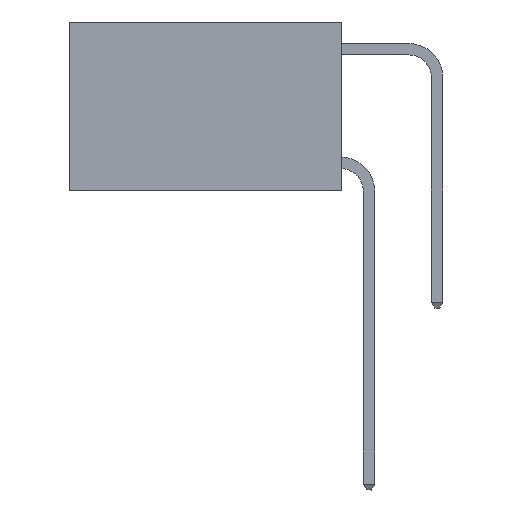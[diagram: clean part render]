
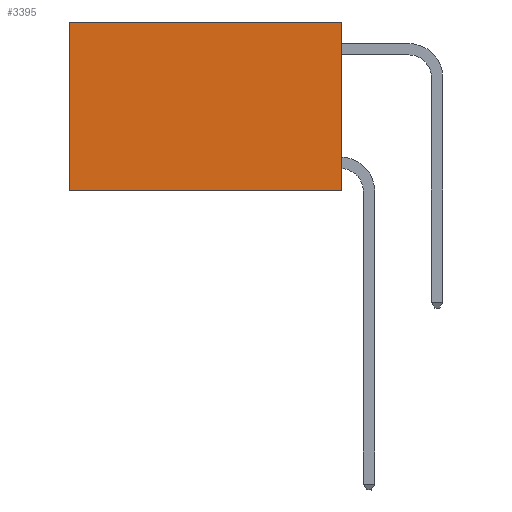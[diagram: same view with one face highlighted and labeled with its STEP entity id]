
A CAD part, left-side view. The second image highlights one B-rep face of the part: STEP entity #3395.
In plain terms, the highlighted planar face has unit normal (-1, 0, 0).
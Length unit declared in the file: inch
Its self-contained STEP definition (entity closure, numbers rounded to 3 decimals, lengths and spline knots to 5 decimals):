
#1128 = VERTEX_POINT ( 'NONE', #1516 ) ;
#1346 = CARTESIAN_POINT ( 'NONE',  ( 0.2625, 0., 0. ) ) ;
#1516 = CARTESIAN_POINT ( 'NONE',  ( 0.2625, 0., 0. ) ) ;
#2384 = VECTOR ( 'NONE', #17193, 39.37008 ) ;
#2615 = CARTESIAN_POINT ( 'NONE',  ( 0.2625, 0., 0. ) ) ;
#3347 = EDGE_CURVE ( 'NONE', #1128, #20527, #14699, .T. ) ;
#3395 = ADVANCED_FACE ( 'NONE', ( #26808 ), #17297, .F. ) ;
#3631 = CARTESIAN_POINT ( 'NONE',  ( 0.2625, 0., -0.37 ) ) ;
#3874 = DIRECTION ( 'NONE',  ( 0., 1., 0. ) ) ;
#5116 = DIRECTION ( 'NONE',  ( 0., 0., -1. ) ) ;
#5907 = DIRECTION ( 'NONE',  ( 0., 0., -1. ) ) ;
#7393 = CARTESIAN_POINT ( 'NONE',  ( 0.2625, 0., 0. ) ) ;
#7721 = CARTESIAN_POINT ( 'NONE',  ( 0.2625, 0., -0.37 ) ) ;
#12131 = LINE ( 'NONE', #3631, #24266 ) ;
#13669 = LINE ( 'NONE', #20490, #20844 ) ;
#14699 = LINE ( 'NONE', #7393, #2384 ) ;
#17193 = DIRECTION ( 'NONE',  ( 0., 0., -1. ) ) ;
#17195 = VECTOR ( 'NONE', #3874, 39.37008 ) ;
#17297 = PLANE ( 'NONE',  #27599 ) ;
#18603 = ORIENTED_EDGE ( 'NONE', *, *, #22784, .T. ) ;
#19708 = ORIENTED_EDGE ( 'NONE', *, *, #22869, .F. ) ;
#19724 = DIRECTION ( 'NONE',  ( 1., 0., 0. ) ) ;
#20490 = CARTESIAN_POINT ( 'NONE',  ( 0.2625, 0.6, 0. ) ) ;
#20527 = VERTEX_POINT ( 'NONE', #7721 ) ;
#20705 = DIRECTION ( 'NONE',  ( 0., 1., 0. ) ) ;
#20844 = VECTOR ( 'NONE', #5907, 39.37008 ) ;
#22183 = VERTEX_POINT ( 'NONE', #25418 ) ;
#22784 = EDGE_CURVE ( 'NONE', #26235, #22183, #13669, .T. ) ;
#22839 = ORIENTED_EDGE ( 'NONE', *, *, #3347, .F. ) ;
#22869 = EDGE_CURVE ( 'NONE', #20527, #22183, #12131, .T. ) ;
#24266 = VECTOR ( 'NONE', #20705, 39.37008 ) ;
#25418 = CARTESIAN_POINT ( 'NONE',  ( 0.2625, 0.6, -0.37 ) ) ;
#26235 = VERTEX_POINT ( 'NONE', #30377 ) ;
#26808 = FACE_OUTER_BOUND ( 'NONE', #29520, .T. ) ;
#27078 = ORIENTED_EDGE ( 'NONE', *, *, #30867, .T. ) ;
#27599 = AXIS2_PLACEMENT_3D ( 'NONE', #2615, #19724, #5116 ) ;
#29520 = EDGE_LOOP ( 'NONE', ( #18603, #19708, #22839, #27078 ) ) ;
#29982 = LINE ( 'NONE', #1346, #17195 ) ;
#30377 = CARTESIAN_POINT ( 'NONE',  ( 0.2625, 0.6, 0. ) ) ;
#30867 = EDGE_CURVE ( 'NONE', #1128, #26235, #29982, .T. ) ;
